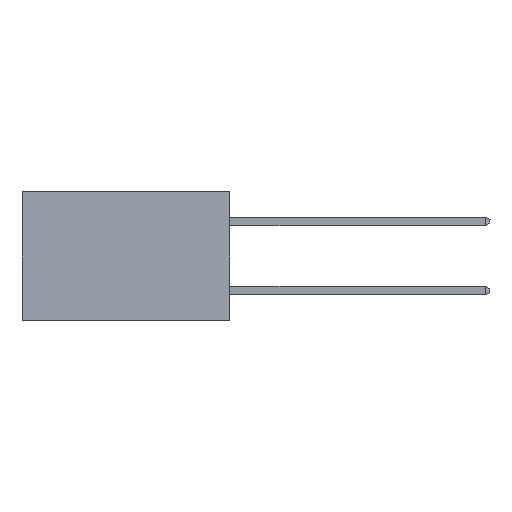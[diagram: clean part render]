
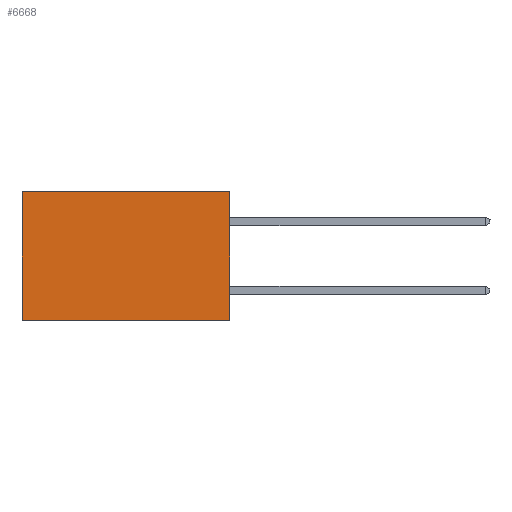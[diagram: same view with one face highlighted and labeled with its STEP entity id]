
A CAD part, left-side view. The second image highlights one B-rep face of the part: STEP entity #6668.
In plain terms, the highlighted planar face has unit normal (-1, 0, 0).
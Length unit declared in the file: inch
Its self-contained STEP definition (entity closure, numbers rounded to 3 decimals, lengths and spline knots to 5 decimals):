
#17 = VERTEX_POINT ( 'NONE', #18031 ) ;
#204 = PLANE ( 'NONE',  #18299 ) ;
#411 = CARTESIAN_POINT ( 'NONE',  ( 0.2615, 0.6, -0.37 ) ) ;
#854 = DIRECTION ( 'NONE',  ( 0., 1., 0. ) ) ;
#1569 = VECTOR ( 'NONE', #854, 39.37008 ) ;
#1732 = EDGE_CURVE ( 'NONE', #17, #4868, #19797, .T. ) ;
#2332 = VECTOR ( 'NONE', #6697, 39.37008 ) ;
#2478 = EDGE_LOOP ( 'NONE', ( #11556, #5710, #9402, #17782 ) ) ;
#4706 = CARTESIAN_POINT ( 'NONE',  ( 0.2615, 0., -0.37 ) ) ;
#4868 = VERTEX_POINT ( 'NONE', #8473 ) ;
#5710 = ORIENTED_EDGE ( 'NONE', *, *, #20110, .F. ) ;
#6556 = DIRECTION ( 'NONE',  ( 0., 0., -1. ) ) ;
#6668 = ADVANCED_FACE ( 'NONE', ( #13136 ), #204, .F. ) ;
#6697 = DIRECTION ( 'NONE',  ( 0., 1., 0. ) ) ;
#7067 = VERTEX_POINT ( 'NONE', #18593 ) ;
#8128 = DIRECTION ( 'NONE',  ( 0., 0., -1. ) ) ;
#8273 = DIRECTION ( 'NONE',  ( 0., 0., -1. ) ) ;
#8473 = CARTESIAN_POINT ( 'NONE',  ( 0.2615, 0.6, -0.37 ) ) ;
#8591 = LINE ( 'NONE', #13376, #17763 ) ;
#9010 = CARTESIAN_POINT ( 'NONE',  ( 0.2615, 0., -0.37 ) ) ;
#9402 = ORIENTED_EDGE ( 'NONE', *, *, #19047, .F. ) ;
#11556 = ORIENTED_EDGE ( 'NONE', *, *, #1732, .T. ) ;
#11796 = CARTESIAN_POINT ( 'NONE',  ( 0.2615, 0., 0. ) ) ;
#12936 = VECTOR ( 'NONE', #8128, 39.37008 ) ;
#13136 = FACE_OUTER_BOUND ( 'NONE', #2478, .T. ) ;
#13376 = CARTESIAN_POINT ( 'NONE',  ( 0.2615, 0., -0.37 ) ) ;
#16553 = LINE ( 'NONE', #9010, #1569 ) ;
#16630 = DIRECTION ( 'NONE',  ( 1., 0., 0. ) ) ;
#16658 = LINE ( 'NONE', #11796, #2332 ) ;
#17635 = EDGE_CURVE ( 'NONE', #7067, #17, #16658, .T. ) ;
#17763 = VECTOR ( 'NONE', #8273, 39.37008 ) ;
#17782 = ORIENTED_EDGE ( 'NONE', *, *, #17635, .T. ) ;
#18031 = CARTESIAN_POINT ( 'NONE',  ( 0.2615, 0.6, 0. ) ) ;
#18107 = CARTESIAN_POINT ( 'NONE',  ( 0.2615, 0., -0.37 ) ) ;
#18299 = AXIS2_PLACEMENT_3D ( 'NONE', #18107, #16630, #6556 ) ;
#18593 = CARTESIAN_POINT ( 'NONE',  ( 0.2615, 0., 0. ) ) ;
#19047 = EDGE_CURVE ( 'NONE', #7067, #19721, #8591, .T. ) ;
#19721 = VERTEX_POINT ( 'NONE', #4706 ) ;
#19797 = LINE ( 'NONE', #411, #12936 ) ;
#20110 = EDGE_CURVE ( 'NONE', #19721, #4868, #16553, .T. ) ;
